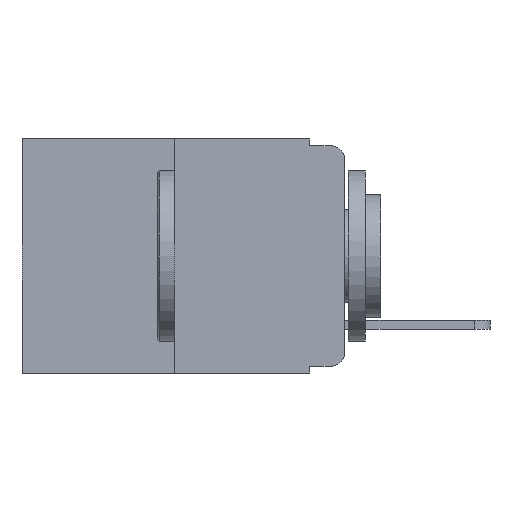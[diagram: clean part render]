
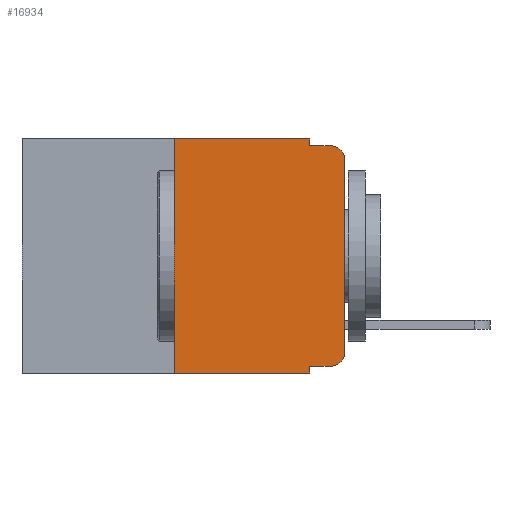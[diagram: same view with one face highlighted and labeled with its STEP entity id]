
A CAD part, left-side view. The second image highlights one B-rep face of the part: STEP entity #16934.
In plain terms, the highlighted planar face has unit normal (-1, 0, 0).
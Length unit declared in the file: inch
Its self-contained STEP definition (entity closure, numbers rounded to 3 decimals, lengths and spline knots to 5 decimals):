
#726 = CARTESIAN_POINT ( 'NONE',  ( 0., 0.02, -0.333 ) ) ;
#957 = VERTEX_POINT ( 'NONE', #726 ) ;
#1352 = LINE ( 'NONE', #11218, #5909 ) ;
#1522 = VECTOR ( 'NONE', #14595, 39.37008 ) ;
#1549 = VECTOR ( 'NONE', #7912, 39.37008 ) ;
#1575 = DIRECTION ( 'NONE',  ( 0., -1., 0. ) ) ;
#1601 = LINE ( 'NONE', #19444, #11695 ) ;
#1644 = ORIENTED_EDGE ( 'NONE', *, *, #9262, .F. ) ;
#1783 = CARTESIAN_POINT ( 'NONE',  ( 0., 0.051, -0.333 ) ) ;
#2156 = DIRECTION ( 'NONE',  ( 1., 0., 0. ) ) ;
#2620 = EDGE_CURVE ( 'NONE', #17552, #9117, #7044, .T. ) ;
#2745 = DIRECTION ( 'NONE',  ( 0., -1., 0. ) ) ;
#3075 = EDGE_CURVE ( 'NONE', #4561, #12313, #1601, .T. ) ;
#3368 = CARTESIAN_POINT ( 'NONE',  ( 0., 0., 0. ) ) ;
#4071 = LINE ( 'NONE', #3368, #1522 ) ;
#4171 = EDGE_CURVE ( 'NONE', #957, #17421, #16958, .T. ) ;
#4328 = VERTEX_POINT ( 'NONE', #17566 ) ;
#4561 = VERTEX_POINT ( 'NONE', #10111 ) ;
#4819 = CARTESIAN_POINT ( 'NONE',  ( 0., 0.051, -0.01 ) ) ;
#5020 = VECTOR ( 'NONE', #15349, 39.37008 ) ;
#5101 = DIRECTION ( 'NONE',  ( 0., 0., -1. ) ) ;
#5162 = VERTEX_POINT ( 'NONE', #14708 ) ;
#5206 = CARTESIAN_POINT ( 'NONE',  ( 0., 0.473, 0. ) ) ;
#5474 = DIRECTION ( 'NONE',  ( -1., 0., 0. ) ) ;
#5497 = LINE ( 'NONE', #14338, #20853 ) ;
#5909 = VECTOR ( 'NONE', #1575, 39.37008 ) ;
#6000 = DIRECTION ( 'NONE',  ( 0., 0., 1. ) ) ;
#6002 = FACE_OUTER_BOUND ( 'NONE', #12963, .T. ) ;
#6029 = CARTESIAN_POINT ( 'NONE',  ( 0., 0., -0.03 ) ) ;
#6278 = DIRECTION ( 'NONE',  ( 0., -1., 0. ) ) ;
#6661 = ORIENTED_EDGE ( 'NONE', *, *, #3075, .F. ) ;
#7003 = DIRECTION ( 'NONE',  ( 0., 0., -1. ) ) ;
#7044 = LINE ( 'NONE', #16906, #5020 ) ;
#7236 = ORIENTED_EDGE ( 'NONE', *, *, #11785, .T. ) ;
#7728 = CARTESIAN_POINT ( 'NONE',  ( 0., 0.051, -0.01 ) ) ;
#7781 = CARTESIAN_POINT ( 'NONE',  ( 0., 0.051, -0.343 ) ) ;
#7912 = DIRECTION ( 'NONE',  ( 0., -1., 0. ) ) ;
#7923 = EDGE_CURVE ( 'NONE', #17552, #957, #8306, .T. ) ;
#8071 = DIRECTION ( 'NONE',  ( -1., 0., 0. ) ) ;
#8214 = CARTESIAN_POINT ( 'NONE',  ( 0., 0., -0.313 ) ) ;
#8306 = LINE ( 'NONE', #15220, #17867 ) ;
#8697 = VERTEX_POINT ( 'NONE', #6029 ) ;
#9117 = VERTEX_POINT ( 'NONE', #7781 ) ;
#9262 = EDGE_CURVE ( 'NONE', #12313, #4328, #15158, .T. ) ;
#9691 = EDGE_CURVE ( 'NONE', #5162, #13948, #18423, .T. ) ;
#10078 = DIRECTION ( 'NONE',  ( 0., 0., -1. ) ) ;
#10111 = CARTESIAN_POINT ( 'NONE',  ( 0., 0.051, 0. ) ) ;
#11218 = CARTESIAN_POINT ( 'NONE',  ( 0., 0.473, 0. ) ) ;
#11460 = ORIENTED_EDGE ( 'NONE', *, *, #17618, .T. ) ;
#11695 = VECTOR ( 'NONE', #10078, 39.37008 ) ;
#11785 = EDGE_CURVE ( 'NONE', #5162, #9117, #5497, .T. ) ;
#11820 = ORIENTED_EDGE ( 'NONE', *, *, #15028, .T. ) ;
#11987 = ORIENTED_EDGE ( 'NONE', *, *, #4171, .T. ) ;
#12313 = VERTEX_POINT ( 'NONE', #7728 ) ;
#12360 = ORIENTED_EDGE ( 'NONE', *, *, #9691, .F. ) ;
#12963 = EDGE_LOOP ( 'NONE', ( #11820, #11460, #1644, #6661, #15249, #12360, #7236, #19477, #16558, #11987 ) ) ;
#13073 = EDGE_CURVE ( 'NONE', #13948, #4561, #1352, .T. ) ;
#13145 = AXIS2_PLACEMENT_3D ( 'NONE', #5206, #2156, #16458 ) ;
#13948 = VERTEX_POINT ( 'NONE', #15138 ) ;
#14338 = CARTESIAN_POINT ( 'NONE',  ( 0., 0.473, -0.343 ) ) ;
#14595 = DIRECTION ( 'NONE',  ( 0., 0., 1. ) ) ;
#14708 = CARTESIAN_POINT ( 'NONE',  ( 0., 0.25, -0.343 ) ) ;
#15028 = EDGE_CURVE ( 'NONE', #17421, #8697, #4071, .T. ) ;
#15138 = CARTESIAN_POINT ( 'NONE',  ( 0., 0.25, 0. ) ) ;
#15158 = LINE ( 'NONE', #4819, #1549 ) ;
#15220 = CARTESIAN_POINT ( 'NONE',  ( 0., 0.051, -0.333 ) ) ;
#15249 = ORIENTED_EDGE ( 'NONE', *, *, #13073, .F. ) ;
#15349 = DIRECTION ( 'NONE',  ( 0., 0., -1. ) ) ;
#15774 = CIRCLE ( 'NONE', #19115, 0.02 ) ;
#16322 = PLANE ( 'NONE',  #13145 ) ;
#16458 = DIRECTION ( 'NONE',  ( 0., 0., -1. ) ) ;
#16558 = ORIENTED_EDGE ( 'NONE', *, *, #7923, .T. ) ;
#16646 = CARTESIAN_POINT ( 'NONE',  ( 0., 0.02, -0.03 ) ) ;
#16906 = CARTESIAN_POINT ( 'NONE',  ( 0., 0.051, 0. ) ) ;
#16934 = ADVANCED_FACE ( 'NONE', ( #6002 ), #16322, .F. ) ;
#16958 = CIRCLE ( 'NONE', #19734, 0.02 ) ;
#17421 = VERTEX_POINT ( 'NONE', #8214 ) ;
#17552 = VERTEX_POINT ( 'NONE', #1783 ) ;
#17566 = CARTESIAN_POINT ( 'NONE',  ( 0., 0.02, -0.01 ) ) ;
#17618 = EDGE_CURVE ( 'NONE', #8697, #4328, #15774, .T. ) ;
#17867 = VECTOR ( 'NONE', #2745, 39.37008 ) ;
#18423 = LINE ( 'NONE', #20227, #19953 ) ;
#19115 = AXIS2_PLACEMENT_3D ( 'NONE', #16646, #5474, #7003 ) ;
#19444 = CARTESIAN_POINT ( 'NONE',  ( 0., 0.051, 0. ) ) ;
#19477 = ORIENTED_EDGE ( 'NONE', *, *, #2620, .F. ) ;
#19734 = AXIS2_PLACEMENT_3D ( 'NONE', #20689, #8071, #5101 ) ;
#19953 = VECTOR ( 'NONE', #6000, 39.37008 ) ;
#20227 = CARTESIAN_POINT ( 'NONE',  ( 0., 0.25, 0. ) ) ;
#20689 = CARTESIAN_POINT ( 'NONE',  ( 0., 0.02, -0.313 ) ) ;
#20853 = VECTOR ( 'NONE', #6278, 39.37008 ) ;
